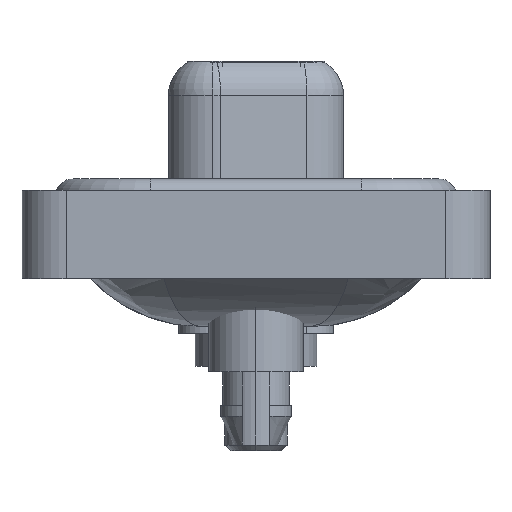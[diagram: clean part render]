
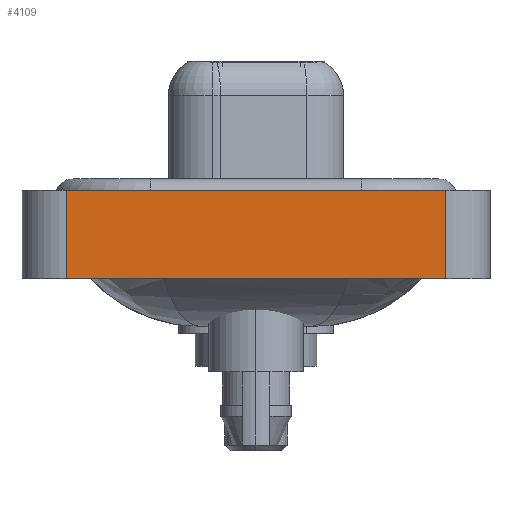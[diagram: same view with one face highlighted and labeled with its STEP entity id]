
A CAD part, left-side view. The second image highlights one B-rep face of the part: STEP entity #4109.
In plain terms, the highlighted planar face has unit normal (-1, 0, 0).
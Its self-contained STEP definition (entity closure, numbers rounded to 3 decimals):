
#200 = CARTESIAN_POINT ( 'NONE',  ( -7.35, -8.55, 0.4 ) ) ;
#372 = LINE ( 'NONE', #200, #2648 ) ;
#1382 = ORIENTED_EDGE ( 'NONE', *, *, #3697, .F. ) ;
#1691 = ORIENTED_EDGE ( 'NONE', *, *, #7040, .T. ) ;
#1756 = VERTEX_POINT ( 'NONE', #5823 ) ;
#2021 = DIRECTION ( 'NONE',  ( 0., 0., 1. ) ) ;
#2648 = VECTOR ( 'NONE', #14963, 1000. ) ;
#3387 = VECTOR ( 'NONE', #14486, 1000. ) ;
#3697 = EDGE_CURVE ( 'NONE', #5656, #1756, #14078, .T. ) ;
#4109 = ADVANCED_FACE ( 'NONE', ( #10806 ), #13441, .T. ) ;
#4652 = ORIENTED_EDGE ( 'NONE', *, *, #6619, .T. ) ;
#4739 = CARTESIAN_POINT ( 'NONE',  ( -7.35, 8.55, -3.6 ) ) ;
#5159 = CARTESIAN_POINT ( 'NONE',  ( -7.35, -8.55, -3.6 ) ) ;
#5180 = DIRECTION ( 'NONE',  ( 0., -1., 0. ) ) ;
#5656 = VERTEX_POINT ( 'NONE', #15001 ) ;
#5721 = CARTESIAN_POINT ( 'NONE',  ( -7.35, -8.55, -3.6 ) ) ;
#5823 = CARTESIAN_POINT ( 'NONE',  ( -7.35, 8.55, 0.4 ) ) ;
#6562 = LINE ( 'NONE', #17227, #14525 ) ;
#6619 = EDGE_CURVE ( 'NONE', #5656, #13212, #6562, .T. ) ;
#6669 = CARTESIAN_POINT ( 'NONE',  ( -7.35, -8.55, 0.4 ) ) ;
#7040 = EDGE_CURVE ( 'NONE', #13212, #10218, #9069, .T. ) ;
#8919 = ORIENTED_EDGE ( 'NONE', *, *, #14782, .F. ) ;
#9069 = LINE ( 'NONE', #5159, #3387 ) ;
#9644 = EDGE_LOOP ( 'NONE', ( #1691, #8919, #1382, #4652 ) ) ;
#10218 = VERTEX_POINT ( 'NONE', #6669 ) ;
#10806 = FACE_OUTER_BOUND ( 'NONE', #9644, .T. ) ;
#10903 = CARTESIAN_POINT ( 'NONE',  ( -7.35, -8.55, -3.6 ) ) ;
#11084 = VECTOR ( 'NONE', #2021, 1000. ) ;
#13212 = VERTEX_POINT ( 'NONE', #5721 ) ;
#13441 = PLANE ( 'NONE',  #14412 ) ;
#14078 = LINE ( 'NONE', #4739, #11084 ) ;
#14412 = AXIS2_PLACEMENT_3D ( 'NONE', #10903, #16156, #16251 ) ;
#14486 = DIRECTION ( 'NONE',  ( 0., 0., 1. ) ) ;
#14525 = VECTOR ( 'NONE', #5180, 1000. ) ;
#14782 = EDGE_CURVE ( 'NONE', #1756, #10218, #372, .T. ) ;
#14963 = DIRECTION ( 'NONE',  ( 0., -1., 0. ) ) ;
#15001 = CARTESIAN_POINT ( 'NONE',  ( -7.35, 8.55, -3.6 ) ) ;
#16156 = DIRECTION ( 'NONE',  ( -1., 0., 0. ) ) ;
#16251 = DIRECTION ( 'NONE',  ( 0., 0., 1. ) ) ;
#17227 = CARTESIAN_POINT ( 'NONE',  ( -7.35, -8.55, -3.6 ) ) ;
